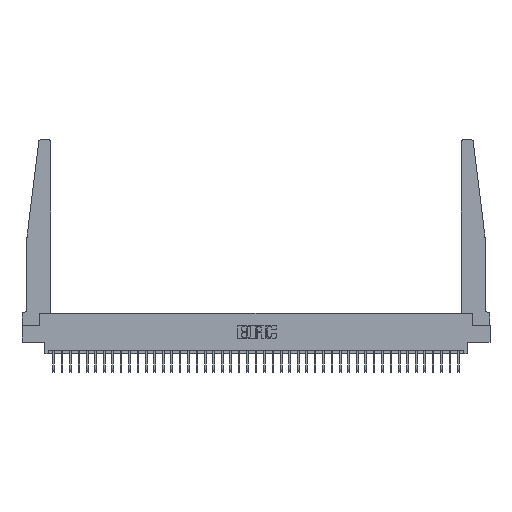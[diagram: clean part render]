
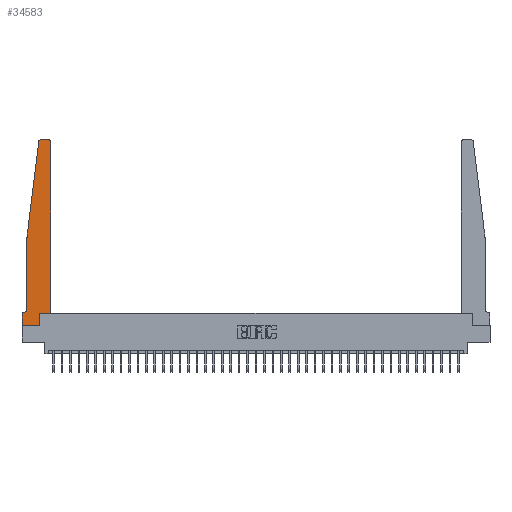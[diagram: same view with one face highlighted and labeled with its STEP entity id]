
A CAD part, top view. The second image highlights one B-rep face of the part: STEP entity #34583.
In plain terms, the highlighted planar face has unit normal (0, 0, 1).
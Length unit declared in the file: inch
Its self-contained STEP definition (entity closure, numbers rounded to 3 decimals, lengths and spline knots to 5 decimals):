
#104 = CARTESIAN_POINT ( 'NONE',  ( 0.2605, 0.18, 0.37 ) ) ;
#433 = VERTEX_POINT ( 'NONE', #34081 ) ;
#727 = VECTOR ( 'NONE', #16610, 39.37008 ) ;
#1422 = ORIENTED_EDGE ( 'NONE', *, *, #23179, .T. ) ;
#1756 = CARTESIAN_POINT ( 'NONE',  ( 0.065, 0.2375, 0.37 ) ) ;
#2025 = DIRECTION ( 'NONE',  ( 0., 0., 1. ) ) ;
#2430 = VERTEX_POINT ( 'NONE', #21018 ) ;
#3150 = DIRECTION ( 'NONE',  ( 0., 1., 0. ) ) ;
#3561 = DIRECTION ( 'NONE',  ( 1., 0., 0. ) ) ;
#4885 = EDGE_CURVE ( 'NONE', #13076, #31109, #10474, .T. ) ;
#5262 = VERTEX_POINT ( 'NONE', #1756 ) ;
#5991 = CARTESIAN_POINT ( 'NONE',  ( 0.425, 2.72, 0.37 ) ) ;
#6740 = LINE ( 'NONE', #33663, #15554 ) ;
#7011 = CARTESIAN_POINT ( 'NONE',  ( 0.395, 2.75, 0.37 ) ) ;
#7028 = DIRECTION ( 'NONE',  ( 1., 0., 0. ) ) ;
#7180 = CARTESIAN_POINT ( 'NONE',  ( 0.27653, 2.72, 0.37 ) ) ;
#7457 = ORIENTED_EDGE ( 'NONE', *, *, #16382, .T. ) ;
#7500 = LINE ( 'NONE', #19434, #727 ) ;
#8038 = EDGE_CURVE ( 'NONE', #433, #29221, #7500, .T. ) ;
#8667 = LINE ( 'NONE', #14435, #15169 ) ;
#8980 = LINE ( 'NONE', #19715, #12767 ) ;
#9294 = CARTESIAN_POINT ( 'NONE',  ( 0.395, 2.72, 0.37 ) ) ;
#10401 = DIRECTION ( 'NONE',  ( 1., 0., 0. ) ) ;
#10421 = EDGE_CURVE ( 'NONE', #2430, #30686, #6740, .T. ) ;
#10474 = LINE ( 'NONE', #18581, #16981 ) ;
#10694 = VERTEX_POINT ( 'NONE', #13375 ) ;
#10791 = ORIENTED_EDGE ( 'NONE', *, *, #8038, .T. ) ;
#10997 = EDGE_CURVE ( 'NONE', #30844, #5262, #8980, .T. ) ;
#11504 = CARTESIAN_POINT ( 'NONE',  ( 0.25, 2.75, 0.37 ) ) ;
#12459 = ORIENTED_EDGE ( 'NONE', *, *, #12584, .T. ) ;
#12584 = EDGE_CURVE ( 'NONE', #29221, #2430, #19503, .T. ) ;
#12644 = VERTEX_POINT ( 'NONE', #7011 ) ;
#12748 = VECTOR ( 'NONE', #3150, 39.37008 ) ;
#12767 = VECTOR ( 'NONE', #23760, 39.37008 ) ;
#12870 = ORIENTED_EDGE ( 'NONE', *, *, #4885, .T. ) ;
#13076 = VERTEX_POINT ( 'NONE', #24909 ) ;
#13269 = CARTESIAN_POINT ( 'NONE',  ( 0.27653, 2.75, 0.37 ) ) ;
#13375 = CARTESIAN_POINT ( 'NONE',  ( 0.24675, 2.72367, 0.37 ) ) ;
#13918 = DIRECTION ( 'NONE',  ( 1., 0., 0. ) ) ;
#14435 = CARTESIAN_POINT ( 'NONE',  ( 0.425, 0.18, 0.37 ) ) ;
#14522 = AXIS2_PLACEMENT_3D ( 'NONE', #21688, #34569, #10401 ) ;
#14807 = VERTEX_POINT ( 'NONE', #104 ) ;
#15108 = ORIENTED_EDGE ( 'NONE', *, *, #26298, .T. ) ;
#15141 = DIRECTION ( 'NONE',  ( 0., 0., -1. ) ) ;
#15169 = VECTOR ( 'NONE', #13918, 39.37008 ) ;
#15554 = VECTOR ( 'NONE', #3561, 39.37008 ) ;
#15685 = CARTESIAN_POINT ( 'NONE',  ( 0.065, 1.25, 0.37 ) ) ;
#15784 = DIRECTION ( 'NONE',  ( 0., 1., 0. ) ) ;
#16228 = ORIENTED_EDGE ( 'NONE', *, *, #10421, .T. ) ;
#16246 = VECTOR ( 'NONE', #17953, 39.37008 ) ;
#16382 = EDGE_CURVE ( 'NONE', #31859, #10694, #25455, .T. ) ;
#16610 = DIRECTION ( 'NONE',  ( -1., 0., 0. ) ) ;
#16788 = LINE ( 'NONE', #11504, #27242 ) ;
#16859 = CARTESIAN_POINT ( 'NONE',  ( 0., 0., 0.37 ) ) ;
#16981 = VECTOR ( 'NONE', #15784, 39.37008 ) ;
#17914 = DIRECTION ( 'NONE',  ( 1., 0., 0. ) ) ;
#17953 = DIRECTION ( 'NONE',  ( -0.122, -0.992, 0. ) ) ;
#17998 = CIRCLE ( 'NONE', #23635, 0.05 ) ;
#18581 = CARTESIAN_POINT ( 'NONE',  ( 0.425, 0.18, 0.37 ) ) ;
#18665 = CARTESIAN_POINT ( 'NONE',  ( 0.2605, 0.18, 0.37 ) ) ;
#18847 = FACE_OUTER_BOUND ( 'NONE', #26363, .T. ) ;
#19434 = CARTESIAN_POINT ( 'NONE',  ( 0.065, 0.1875, 0.37 ) ) ;
#19503 = LINE ( 'NONE', #16859, #32486 ) ;
#19715 = CARTESIAN_POINT ( 'NONE',  ( 0.065, 1.25, 0.37 ) ) ;
#20069 = CARTESIAN_POINT ( 'NONE',  ( 0.065, 1.25, 0.37 ) ) ;
#20838 = ORIENTED_EDGE ( 'NONE', *, *, #26474, .T. ) ;
#20979 = DIRECTION ( 'NONE',  ( -1., 0., 0. ) ) ;
#21018 = CARTESIAN_POINT ( 'NONE',  ( 0., 0., 0.37 ) ) ;
#21261 = EDGE_CURVE ( 'NONE', #12644, #31859, #16788, .T. ) ;
#21688 = CARTESIAN_POINT ( 'NONE',  ( 0., 0.1875, 0.37 ) ) ;
#22332 = DIRECTION ( 'NONE',  ( 0., -1., 0. ) ) ;
#22561 = CARTESIAN_POINT ( 'NONE',  ( 0.2605, 0., 0.37 ) ) ;
#22684 = DIRECTION ( 'NONE',  ( 0., 0., 1. ) ) ;
#23076 = CARTESIAN_POINT ( 'NONE',  ( 0.015, 0.2375, 0.37 ) ) ;
#23179 = EDGE_CURVE ( 'NONE', #30686, #14807, #29432, .T. ) ;
#23635 = AXIS2_PLACEMENT_3D ( 'NONE', #23076, #15141, #20979 ) ;
#23760 = DIRECTION ( 'NONE',  ( 0., -1., 0. ) ) ;
#24356 = CARTESIAN_POINT ( 'NONE',  ( 0., 0.1875, 0.37 ) ) ;
#24909 = CARTESIAN_POINT ( 'NONE',  ( 0.425, 0.18, 0.37 ) ) ;
#25455 = CIRCLE ( 'NONE', #28305, 0.03 ) ;
#25577 = EDGE_CURVE ( 'NONE', #31109, #12644, #26953, .T. ) ;
#26298 = EDGE_CURVE ( 'NONE', #14807, #13076, #8667, .T. ) ;
#26363 = EDGE_LOOP ( 'NONE', ( #32108, #7457, #32398, #32671, #20838, #10791, #12459, #16228, #1422, #15108, #12870, #34353 ) ) ;
#26474 = EDGE_CURVE ( 'NONE', #5262, #433, #17998, .T. ) ;
#26953 = CIRCLE ( 'NONE', #30899, 0.03 ) ;
#27242 = VECTOR ( 'NONE', #33018, 39.37008 ) ;
#28177 = LINE ( 'NONE', #20069, #16246 ) ;
#28305 = AXIS2_PLACEMENT_3D ( 'NONE', #7180, #2025, #17914 ) ;
#29221 = VERTEX_POINT ( 'NONE', #24356 ) ;
#29273 = PLANE ( 'NONE',  #14522 ) ;
#29432 = LINE ( 'NONE', #18665, #12748 ) ;
#30686 = VERTEX_POINT ( 'NONE', #22561 ) ;
#30844 = VERTEX_POINT ( 'NONE', #15685 ) ;
#30899 = AXIS2_PLACEMENT_3D ( 'NONE', #9294, #22684, #7028 ) ;
#31109 = VERTEX_POINT ( 'NONE', #5991 ) ;
#31859 = VERTEX_POINT ( 'NONE', #13269 ) ;
#32108 = ORIENTED_EDGE ( 'NONE', *, *, #21261, .T. ) ;
#32398 = ORIENTED_EDGE ( 'NONE', *, *, #34808, .T. ) ;
#32486 = VECTOR ( 'NONE', #22332, 39.37008 ) ;
#32671 = ORIENTED_EDGE ( 'NONE', *, *, #10997, .T. ) ;
#33018 = DIRECTION ( 'NONE',  ( -1., 0., 0. ) ) ;
#33663 = CARTESIAN_POINT ( 'NONE',  ( 0., 0., 0.37 ) ) ;
#34081 = CARTESIAN_POINT ( 'NONE',  ( 0.015, 0.1875, 0.37 ) ) ;
#34353 = ORIENTED_EDGE ( 'NONE', *, *, #25577, .T. ) ;
#34569 = DIRECTION ( 'NONE',  ( 0., 0., 1. ) ) ;
#34583 = ADVANCED_FACE ( 'NONE', ( #18847 ), #29273, .T. ) ;
#34808 = EDGE_CURVE ( 'NONE', #10694, #30844, #28177, .T. ) ;
